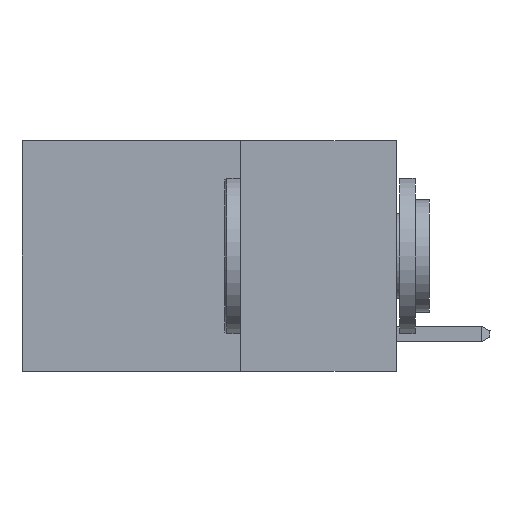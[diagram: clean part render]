
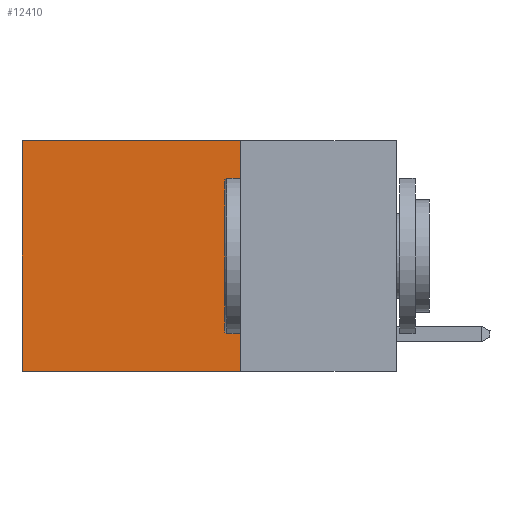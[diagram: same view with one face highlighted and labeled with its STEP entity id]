
A CAD part, left-side view. The second image highlights one B-rep face of the part: STEP entity #12410.
In plain terms, the highlighted planar face has unit normal (-1, 0, 0).
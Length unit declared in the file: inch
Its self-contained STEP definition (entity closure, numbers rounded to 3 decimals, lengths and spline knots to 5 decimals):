
#1188 = CARTESIAN_POINT ( 'NONE',  ( 0.2625, 0.6, 0. ) ) ;
#3751 = DIRECTION ( 'NONE',  ( 0., 0., -1. ) ) ;
#5056 = LINE ( 'NONE', #1188, #13851 ) ;
#5185 = LINE ( 'NONE', #21685, #5459 ) ;
#5306 = DIRECTION ( 'NONE',  ( 0., 1., 0. ) ) ;
#5459 = VECTOR ( 'NONE', #5306, 39.37008 ) ;
#5954 = ORIENTED_EDGE ( 'NONE', *, *, #11484, .T. ) ;
#6698 = VECTOR ( 'NONE', #12135, 39.37008 ) ;
#6817 = VERTEX_POINT ( 'NONE', #11523 ) ;
#8299 = CARTESIAN_POINT ( 'NONE',  ( 0.2625, 0.6, -0.37 ) ) ;
#9879 = EDGE_CURVE ( 'NONE', #14167, #11321, #20776, .T. ) ;
#10035 = CARTESIAN_POINT ( 'NONE',  ( 0.2625, 0.25, 0. ) ) ;
#10099 = CARTESIAN_POINT ( 'NONE',  ( 0.2625, 0.25, -0.37 ) ) ;
#10108 = EDGE_CURVE ( 'NONE', #10790, #14167, #12918, .T. ) ;
#10279 = CARTESIAN_POINT ( 'NONE',  ( 0.2625, 0.25, -0.37 ) ) ;
#10790 = VERTEX_POINT ( 'NONE', #13663 ) ;
#11321 = VERTEX_POINT ( 'NONE', #8299 ) ;
#11484 = EDGE_CURVE ( 'NONE', #10790, #6817, #5185, .T. ) ;
#11523 = CARTESIAN_POINT ( 'NONE',  ( 0.2625, 0.6, 0. ) ) ;
#11673 = AXIS2_PLACEMENT_3D ( 'NONE', #10035, #11833, #12070 ) ;
#11833 = DIRECTION ( 'NONE',  ( 1., 0., 0. ) ) ;
#12070 = DIRECTION ( 'NONE',  ( 0., 0., -1. ) ) ;
#12135 = DIRECTION ( 'NONE',  ( 0., 1., 0. ) ) ;
#12410 = ADVANCED_FACE ( 'NONE', ( #13071 ), #17906, .F. ) ;
#12675 = ORIENTED_EDGE ( 'NONE', *, *, #9879, .F. ) ;
#12918 = LINE ( 'NONE', #16195, #21888 ) ;
#13071 = FACE_OUTER_BOUND ( 'NONE', #14996, .T. ) ;
#13663 = CARTESIAN_POINT ( 'NONE',  ( 0.2625, 0.25, 0. ) ) ;
#13851 = VECTOR ( 'NONE', #22594, 39.37008 ) ;
#14167 = VERTEX_POINT ( 'NONE', #10279 ) ;
#14484 = EDGE_CURVE ( 'NONE', #6817, #11321, #5056, .T. ) ;
#14996 = EDGE_LOOP ( 'NONE', ( #15551, #12675, #16456, #5954 ) ) ;
#15551 = ORIENTED_EDGE ( 'NONE', *, *, #14484, .T. ) ;
#16195 = CARTESIAN_POINT ( 'NONE',  ( 0.2625, 0.25, 0. ) ) ;
#16456 = ORIENTED_EDGE ( 'NONE', *, *, #10108, .F. ) ;
#17906 = PLANE ( 'NONE',  #11673 ) ;
#20776 = LINE ( 'NONE', #10099, #6698 ) ;
#21685 = CARTESIAN_POINT ( 'NONE',  ( 0.2625, 0.25, 0. ) ) ;
#21888 = VECTOR ( 'NONE', #3751, 39.37008 ) ;
#22594 = DIRECTION ( 'NONE',  ( 0., 0., -1. ) ) ;
